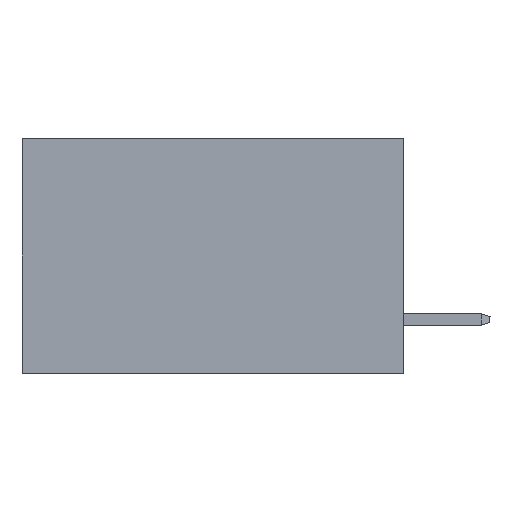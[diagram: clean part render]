
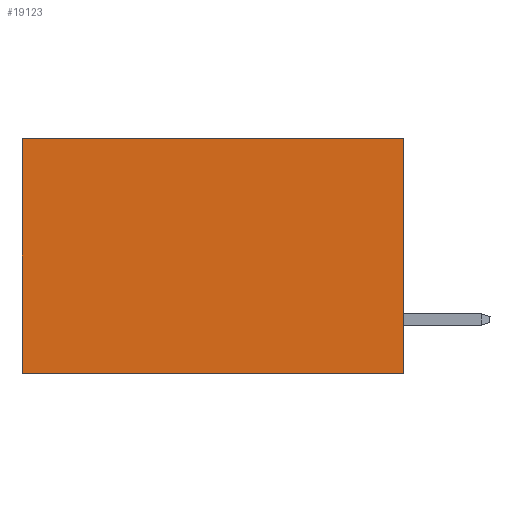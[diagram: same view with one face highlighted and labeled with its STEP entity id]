
A CAD part, left-side view. The second image highlights one B-rep face of the part: STEP entity #19123.
In plain terms, the highlighted planar face has unit normal (-1, 0, 0).
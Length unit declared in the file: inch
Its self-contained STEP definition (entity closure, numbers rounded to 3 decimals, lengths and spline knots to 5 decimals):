
#231 = EDGE_CURVE ( 'NONE', #12243, #3802, #16649, .T. ) ;
#517 = VECTOR ( 'NONE', #20924, 39.37008 ) ;
#2450 = ORIENTED_EDGE ( 'NONE', *, *, #11597, .T. ) ;
#3802 = VERTEX_POINT ( 'NONE', #15462 ) ;
#3932 = LINE ( 'NONE', #9758, #10314 ) ;
#4580 = ORIENTED_EDGE ( 'NONE', *, *, #22719, .F. ) ;
#4986 = EDGE_CURVE ( 'NONE', #16358, #3802, #5613, .T. ) ;
#5613 = LINE ( 'NONE', #18983, #517 ) ;
#6355 = AXIS2_PLACEMENT_3D ( 'NONE', #23369, #6736, #21550 ) ;
#6405 = CARTESIAN_POINT ( 'NONE',  ( 0.2875, 0.6, 0. ) ) ;
#6736 = DIRECTION ( 'NONE',  ( 1., 0., 0. ) ) ;
#7178 = DIRECTION ( 'NONE',  ( 0., 1., 0. ) ) ;
#8569 = FACE_OUTER_BOUND ( 'NONE', #23783, .T. ) ;
#9011 = CARTESIAN_POINT ( 'NONE',  ( 0.2875, 0., -0.37 ) ) ;
#9758 = CARTESIAN_POINT ( 'NONE',  ( 0.2875, 0., 0. ) ) ;
#10314 = VECTOR ( 'NONE', #17165, 39.37008 ) ;
#10829 = CARTESIAN_POINT ( 'NONE',  ( 0.2875, 0., 0. ) ) ;
#11355 = VERTEX_POINT ( 'NONE', #10829 ) ;
#11597 = EDGE_CURVE ( 'NONE', #11355, #16358, #11776, .T. ) ;
#11776 = LINE ( 'NONE', #15554, #14661 ) ;
#12243 = VERTEX_POINT ( 'NONE', #13055 ) ;
#13055 = CARTESIAN_POINT ( 'NONE',  ( 0.2875, 0., -0.37 ) ) ;
#13771 = VECTOR ( 'NONE', #7178, 39.37008 ) ;
#14248 = ORIENTED_EDGE ( 'NONE', *, *, #4986, .T. ) ;
#14661 = VECTOR ( 'NONE', #19438, 39.37008 ) ;
#15462 = CARTESIAN_POINT ( 'NONE',  ( 0.2875, 0.6, -0.37 ) ) ;
#15554 = CARTESIAN_POINT ( 'NONE',  ( 0.2875, 0., 0. ) ) ;
#15980 = PLANE ( 'NONE',  #6355 ) ;
#16358 = VERTEX_POINT ( 'NONE', #6405 ) ;
#16649 = LINE ( 'NONE', #9011, #13771 ) ;
#17165 = DIRECTION ( 'NONE',  ( 0., 0., -1. ) ) ;
#18983 = CARTESIAN_POINT ( 'NONE',  ( 0.2875, 0.6, 0. ) ) ;
#19123 = ADVANCED_FACE ( 'NONE', ( #8569 ), #15980, .F. ) ;
#19438 = DIRECTION ( 'NONE',  ( 0., 1., 0. ) ) ;
#20924 = DIRECTION ( 'NONE',  ( 0., 0., -1. ) ) ;
#21550 = DIRECTION ( 'NONE',  ( 0., 0., -1. ) ) ;
#21824 = ORIENTED_EDGE ( 'NONE', *, *, #231, .F. ) ;
#22719 = EDGE_CURVE ( 'NONE', #11355, #12243, #3932, .T. ) ;
#23369 = CARTESIAN_POINT ( 'NONE',  ( 0.2875, 0., 0. ) ) ;
#23783 = EDGE_LOOP ( 'NONE', ( #14248, #21824, #4580, #2450 ) ) ;
